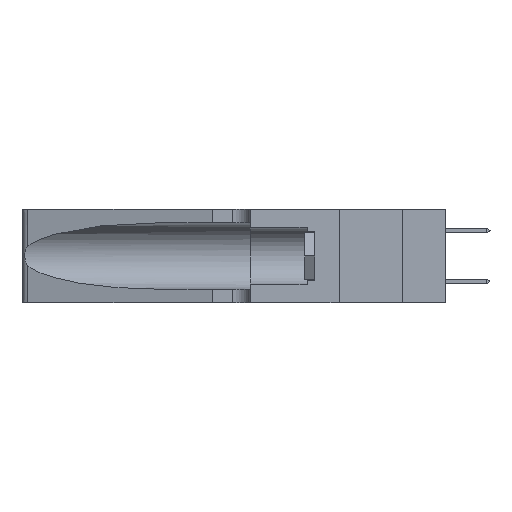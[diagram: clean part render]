
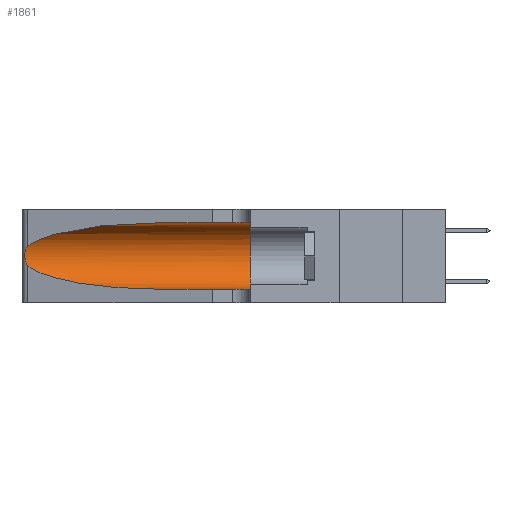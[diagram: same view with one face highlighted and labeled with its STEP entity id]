
A CAD part, left-side view. The second image highlights one B-rep face of the part: STEP entity #1861.
In plain terms, the highlighted cylindrical face has radius 3.308 mm (diameter 6.617 mm), a partial arc.
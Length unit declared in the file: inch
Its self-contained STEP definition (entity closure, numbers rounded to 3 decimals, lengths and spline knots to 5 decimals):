
#1005 = AXIS2_PLACEMENT_3D ( 'NONE', #29414, #39391, #20077 ) ;
#1091 = CARTESIAN_POINT ( 'NONE',  ( 0.1305, 0.72297, 0.31525 ) ) ;
#1209 = CARTESIAN_POINT ( 'NONE',  ( 0.1305, 0.72297, 0.05475 ) ) ;
#1861 = ADVANCED_FACE ( 'NONE', ( #3239 ), #30201, .F. ) ;
#1964 = CARTESIAN_POINT ( 'NONE',  ( 0.25487, 1.22718, 0.22369 ) ) ;
#2035 = CARTESIAN_POINT ( 'NONE',  ( 0.2373, 1.15595, 0.08982 ) ) ;
#2121 = ORIENTED_EDGE ( 'NONE', *, *, #23755, .F. ) ;
#2214 = CARTESIAN_POINT ( 'NONE',  ( 0.1305, 0.35, 0.05475 ) ) ;
#2224 = EDGE_CURVE ( 'NONE', #13773, #22224, #17717, .T. ) ;
#3134 = DIRECTION ( 'NONE',  ( 0., -1., 0. ) ) ;
#3239 = FACE_OUTER_BOUND ( 'NONE', #28283, .T. ) ;
#5227 = EDGE_CURVE ( 'NONE', #13773, #19320, #21632, .T. ) ;
#7127 = EDGE_CURVE ( 'NONE', #21090, #38696, #37711, .T. ) ;
#7308 = CARTESIAN_POINT ( 'NONE',  ( 0.1305, 0.35, 0.31525 ) ) ;
#7537 = DIRECTION ( 'NONE',  ( 0., -1., 0. ) ) ;
#8577 = CARTESIAN_POINT ( 'NONE',  ( 0.25854, 1.2359, 0.20912 ) ) ;
#8712 = CARTESIAN_POINT ( 'NONE',  ( 0.25555, 1.22993, 0.14849 ) ) ;
#10435 = CARTESIAN_POINT ( 'NONE',  ( 0.1305, 0.72297, 0.31525 ) ) ;
#10769 = CARTESIAN_POINT ( 'NONE',  ( 0.2373, 1.15595, 0.28018 ) ) ;
#11789 = CARTESIAN_POINT ( 'NONE',  ( 0.25789, 1.23486, 0.15765 ) ) ;
#11923 = CARTESIAN_POINT ( 'NONE',  ( 0.25639, 1.23186, 0.15144 ) ) ;
#12355 = CIRCLE ( 'NONE', #30888, 0.13025 ) ;
#12590 = ORIENTED_EDGE ( 'NONE', *, *, #40860, .T. ) ;
#13773 = VERTEX_POINT ( 'NONE', #10435 ) ;
#14733 = CARTESIAN_POINT ( 'NONE',  ( 0.25639, 1.23184, 0.21858 ) ) ;
#14760 = VECTOR ( 'NONE', #3134, 39.37008 ) ;
#14848 = CARTESIAN_POINT ( 'NONE',  ( 0.25487, 1.22718, 0.14631 ) ) ;
#15496 = CARTESIAN_POINT ( 'NONE',  ( 0.1305, 1.61858, 0.31525 ) ) ;
#17271 = B_SPLINE_CURVE_WITH_KNOTS ( 'NONE', 3,
 ( #1964, #30981, #14733, #40667, #8577, #30848, #18446, #21652, #27795, #18310, #11789, #11923, #8712, #30723 ),
 .UNSPECIFIED., .F., .F.,
 ( 4, 2, 2, 2, 2, 2, 4 ),
 ( 0., 0.00027, 0.00053, 0.00107, 0.0016, 0.00187, 0.00214 ),
 .UNSPECIFIED. ) ;
#17717 = LINE ( 'NONE', #15496, #14760 ) ;
#18310 = CARTESIAN_POINT ( 'NONE',  ( 0.25856, 1.23593, 0.16098 ) ) ;
#18446 = CARTESIAN_POINT ( 'NONE',  ( 0.26075, 1.23896, 0.19203 ) ) ;
#19320 = VERTEX_POINT ( 'NONE', #33814 ) ;
#20077 = DIRECTION ( 'NONE',  ( 0., 0., -1. ) ) ;
#21023 = CARTESIAN_POINT ( 'NONE',  ( 0.18966, 0.96281, 0.05475 ) ) ;
#21090 = VERTEX_POINT ( 'NONE', #1209 ) ;
#21141 = DIRECTION ( 'NONE',  ( 0., 1., 0. ) ) ;
#21632 =( BOUNDED_CURVE ( )  B_SPLINE_CURVE ( 3, ( #1091, #29845, #10769, #39396 ),
 .UNSPECIFIED., .F., .T. ) 
 B_SPLINE_CURVE_WITH_KNOTS ( ( 4, 4 ),
 ( 1.5708, 2.84003 ),
 .UNSPECIFIED. ) 
 CURVE ( )  GEOMETRIC_REPRESENTATION_ITEM ( )  RATIONAL_B_SPLINE_CURVE ( ( 1., 0.87, 0.87, 1. ) ) 
 REPRESENTATION_ITEM ( '' )  );
#21652 = CARTESIAN_POINT ( 'NONE',  ( 0.26075, 1.23896, 0.178 ) ) ;
#22224 = VERTEX_POINT ( 'NONE', #7308 ) ;
#23755 = EDGE_CURVE ( 'NONE', #22224, #38696, #12355, .T. ) ;
#24368 = DIRECTION ( 'NONE',  ( 0., 0., 1. ) ) ;
#24604 = ORIENTED_EDGE ( 'NONE', *, *, #7127, .T. ) ;
#24614 = VERTEX_POINT ( 'NONE', #14848 ) ;
#25248 = EDGE_CURVE ( 'NONE', #24614, #21090, #28302, .T. ) ;
#25537 = ORIENTED_EDGE ( 'NONE', *, *, #2224, .F. ) ;
#27177 = CARTESIAN_POINT ( 'NONE',  ( 0.1305, 0.72297, 0.05475 ) ) ;
#27425 = CARTESIAN_POINT ( 'NONE',  ( 0.1305, 0.35, 0.185 ) ) ;
#27795 = CARTESIAN_POINT ( 'NONE',  ( 0.26017, 1.23833, 0.17102 ) ) ;
#28189 = ORIENTED_EDGE ( 'NONE', *, *, #5227, .T. ) ;
#28283 = EDGE_LOOP ( 'NONE', ( #28189, #12590, #37062, #24604, #2121, #25537 ) ) ;
#28302 =( BOUNDED_CURVE ( )  B_SPLINE_CURVE ( 3, ( #40326, #2035, #21023, #27177 ),
 .UNSPECIFIED., .F., .F. ) 
 B_SPLINE_CURVE_WITH_KNOTS ( ( 4, 4 ),
 ( 3.44316, 4.71239 ),
 .UNSPECIFIED. ) 
 CURVE ( )  GEOMETRIC_REPRESENTATION_ITEM ( )  RATIONAL_B_SPLINE_CURVE ( ( 1., 0.87, 0.87, 1. ) ) 
 REPRESENTATION_ITEM ( '' )  );
#29414 = CARTESIAN_POINT ( 'NONE',  ( 0.1305, 1.61858, 0.185 ) ) ;
#29549 = CARTESIAN_POINT ( 'NONE',  ( 0.1305, 1.61858, 0.05475 ) ) ;
#29845 = CARTESIAN_POINT ( 'NONE',  ( 0.18966, 0.96281, 0.31525 ) ) ;
#30201 = CYLINDRICAL_SURFACE ( 'NONE', #1005, 0.13025 ) ;
#30723 = CARTESIAN_POINT ( 'NONE',  ( 0.25487, 1.22718, 0.14631 ) ) ;
#30848 = CARTESIAN_POINT ( 'NONE',  ( 0.26018, 1.23835, 0.19895 ) ) ;
#30888 = AXIS2_PLACEMENT_3D ( 'NONE', #27425, #21141, #24368 ) ;
#30981 = CARTESIAN_POINT ( 'NONE',  ( 0.25555, 1.22994, 0.2215 ) ) ;
#33814 = CARTESIAN_POINT ( 'NONE',  ( 0.25487, 1.22718, 0.22369 ) ) ;
#37062 = ORIENTED_EDGE ( 'NONE', *, *, #25248, .T. ) ;
#37711 = LINE ( 'NONE', #29549, #41163 ) ;
#38696 = VERTEX_POINT ( 'NONE', #2214 ) ;
#39391 = DIRECTION ( 'NONE',  ( 0., -1., 0. ) ) ;
#39396 = CARTESIAN_POINT ( 'NONE',  ( 0.25487, 1.22718, 0.22369 ) ) ;
#40326 = CARTESIAN_POINT ( 'NONE',  ( 0.25487, 1.22718, 0.14631 ) ) ;
#40667 = CARTESIAN_POINT ( 'NONE',  ( 0.25787, 1.23484, 0.2124 ) ) ;
#40860 = EDGE_CURVE ( 'NONE', #19320, #24614, #17271, .T. ) ;
#41163 = VECTOR ( 'NONE', #7537, 39.37008 ) ;
